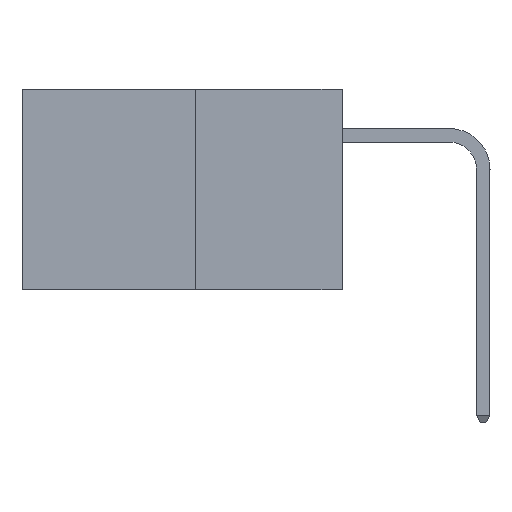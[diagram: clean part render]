
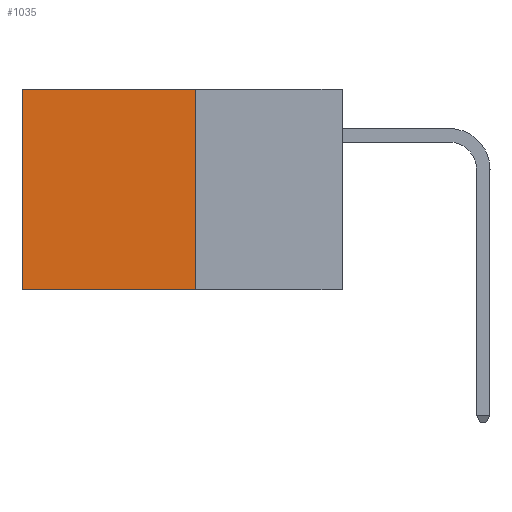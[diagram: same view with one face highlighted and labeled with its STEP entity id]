
A CAD part, left-side view. The second image highlights one B-rep face of the part: STEP entity #1035.
In plain terms, the highlighted planar face has unit normal (-1, 0, 0).
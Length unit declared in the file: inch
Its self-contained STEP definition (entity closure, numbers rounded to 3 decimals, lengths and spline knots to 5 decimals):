
#1035 = ADVANCED_FACE ( 'NONE', ( #18481 ), #22023, .F. ) ;
#1076 = LINE ( 'NONE', #15280, #16759 ) ;
#2458 = EDGE_CURVE ( 'NONE', #4266, #20241, #26713, .T. ) ;
#3916 = EDGE_CURVE ( 'NONE', #10682, #4266, #15667, .T. ) ;
#4266 = VERTEX_POINT ( 'NONE', #21674 ) ;
#4466 = EDGE_CURVE ( 'NONE', #10682, #20877, #22451, .T. ) ;
#4595 = DIRECTION ( 'NONE',  ( 0., 0., -1. ) ) ;
#5264 = DIRECTION ( 'NONE',  ( 0., 0., -1. ) ) ;
#5336 = VECTOR ( 'NONE', #18450, 39.37008 ) ;
#6582 = ORIENTED_EDGE ( 'NONE', *, *, #24998, .T. ) ;
#6737 = CARTESIAN_POINT ( 'NONE',  ( 0.277, 0.27, -0.37 ) ) ;
#9302 = VECTOR ( 'NONE', #5264, 39.37008 ) ;
#9311 = DIRECTION ( 'NONE',  ( 0., 0., -1. ) ) ;
#10682 = VERTEX_POINT ( 'NONE', #11784 ) ;
#11784 = CARTESIAN_POINT ( 'NONE',  ( 0.277, 0.27, 0. ) ) ;
#13170 = DIRECTION ( 'NONE',  ( 1., 0., 0. ) ) ;
#13808 = CARTESIAN_POINT ( 'NONE',  ( 0.277, 0.27, -0.37 ) ) ;
#14361 = CARTESIAN_POINT ( 'NONE',  ( 0.277, 0.27, -0.37 ) ) ;
#15280 = CARTESIAN_POINT ( 'NONE',  ( 0.277, 0.59, -0.37 ) ) ;
#15667 = LINE ( 'NONE', #6737, #9302 ) ;
#15736 = CARTESIAN_POINT ( 'NONE',  ( 0.277, 0.59, 0. ) ) ;
#16759 = VECTOR ( 'NONE', #4595, 39.37008 ) ;
#17554 = ORIENTED_EDGE ( 'NONE', *, *, #2458, .F. ) ;
#18450 = DIRECTION ( 'NONE',  ( 0., 1., 0. ) ) ;
#18481 = FACE_OUTER_BOUND ( 'NONE', #21322, .T. ) ;
#18539 = CARTESIAN_POINT ( 'NONE',  ( 0.277, 0.27, 0. ) ) ;
#18862 = DIRECTION ( 'NONE',  ( 0., 1., 0. ) ) ;
#20241 = VERTEX_POINT ( 'NONE', #22037 ) ;
#20877 = VERTEX_POINT ( 'NONE', #15736 ) ;
#21322 = EDGE_LOOP ( 'NONE', ( #6582, #17554, #23645, #22328 ) ) ;
#21674 = CARTESIAN_POINT ( 'NONE',  ( 0.277, 0.27, -0.37 ) ) ;
#22023 = PLANE ( 'NONE',  #27065 ) ;
#22037 = CARTESIAN_POINT ( 'NONE',  ( 0.277, 0.59, -0.37 ) ) ;
#22328 = ORIENTED_EDGE ( 'NONE', *, *, #4466, .T. ) ;
#22451 = LINE ( 'NONE', #18539, #5336 ) ;
#23645 = ORIENTED_EDGE ( 'NONE', *, *, #3916, .F. ) ;
#24998 = EDGE_CURVE ( 'NONE', #20877, #20241, #1076, .T. ) ;
#25400 = VECTOR ( 'NONE', #18862, 39.37008 ) ;
#26713 = LINE ( 'NONE', #13808, #25400 ) ;
#27065 = AXIS2_PLACEMENT_3D ( 'NONE', #14361, #13170, #9311 ) ;
